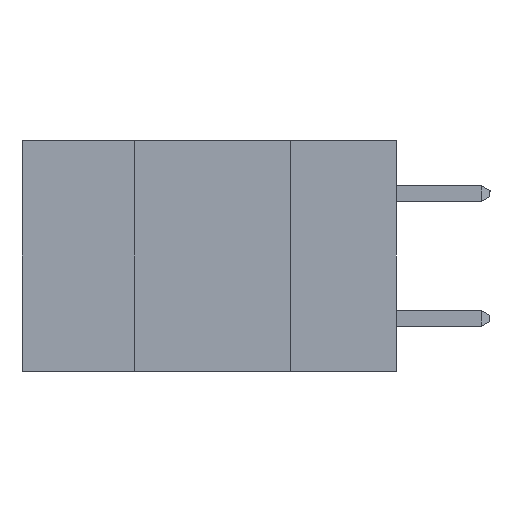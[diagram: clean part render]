
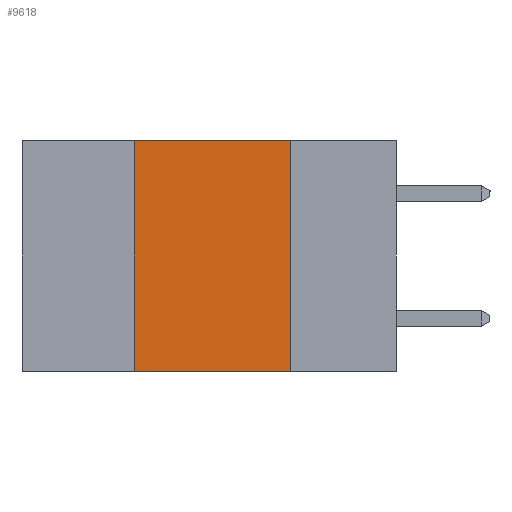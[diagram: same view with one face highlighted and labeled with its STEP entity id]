
A CAD part, left-side view. The second image highlights one B-rep face of the part: STEP entity #9618.
In plain terms, the highlighted planar face has unit normal (-1, 0, 0).
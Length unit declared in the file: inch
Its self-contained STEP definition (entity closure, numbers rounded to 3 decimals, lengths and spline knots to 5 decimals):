
#671 = VERTEX_POINT ( 'NONE', #12134 ) ;
#997 = FACE_OUTER_BOUND ( 'NONE', #4596, .T. ) ;
#1128 = EDGE_CURVE ( 'NONE', #8551, #1817, #10990, .T. ) ;
#1303 = ORIENTED_EDGE ( 'NONE', *, *, #12067, .F. ) ;
#1817 = VERTEX_POINT ( 'NONE', #8210 ) ;
#1913 = VERTEX_POINT ( 'NONE', #12137 ) ;
#2540 = DIRECTION ( 'NONE',  ( 0., 0., -1. ) ) ;
#2556 = EDGE_CURVE ( 'NONE', #671, #1913, #8167, .T. ) ;
#2598 = LINE ( 'NONE', #8309, #9945 ) ;
#4596 = EDGE_LOOP ( 'NONE', ( #7938, #5382, #1303, #8873 ) ) ;
#4763 = DIRECTION ( 'NONE',  ( 0., -1., 0. ) ) ;
#4802 = PLANE ( 'NONE',  #6367 ) ;
#4864 = DIRECTION ( 'NONE',  ( 1., 0., 0. ) ) ;
#5376 = CARTESIAN_POINT ( 'NONE',  ( 0., 0.6, -0.37 ) ) ;
#5382 = ORIENTED_EDGE ( 'NONE', *, *, #1128, .F. ) ;
#6367 = AXIS2_PLACEMENT_3D ( 'NONE', #8585, #4864, #9577 ) ;
#7640 = CARTESIAN_POINT ( 'NONE',  ( 0., 0.42, -0.37 ) ) ;
#7891 = DIRECTION ( 'NONE',  ( 0., 0., 1. ) ) ;
#7938 = ORIENTED_EDGE ( 'NONE', *, *, #10925, .F. ) ;
#8167 = LINE ( 'NONE', #5376, #10808 ) ;
#8210 = CARTESIAN_POINT ( 'NONE',  ( 0., 0.17, 0. ) ) ;
#8309 = CARTESIAN_POINT ( 'NONE',  ( 0., 0.17, -0.37 ) ) ;
#8484 = CARTESIAN_POINT ( 'NONE',  ( 0., 0.6, 0. ) ) ;
#8551 = VERTEX_POINT ( 'NONE', #9122 ) ;
#8585 = CARTESIAN_POINT ( 'NONE',  ( 0., 0.6, 0. ) ) ;
#8816 = LINE ( 'NONE', #7640, #10751 ) ;
#8873 = ORIENTED_EDGE ( 'NONE', *, *, #2556, .T. ) ;
#9122 = CARTESIAN_POINT ( 'NONE',  ( 0., 0.42, 0. ) ) ;
#9518 = VECTOR ( 'NONE', #4763, 39.37008 ) ;
#9577 = DIRECTION ( 'NONE',  ( 0., 0., -1. ) ) ;
#9618 = ADVANCED_FACE ( 'NONE', ( #997 ), #4802, .F. ) ;
#9945 = VECTOR ( 'NONE', #2540, 39.37008 ) ;
#10751 = VECTOR ( 'NONE', #7891, 39.37008 ) ;
#10808 = VECTOR ( 'NONE', #11972, 39.37008 ) ;
#10925 = EDGE_CURVE ( 'NONE', #1817, #1913, #2598, .T. ) ;
#10990 = LINE ( 'NONE', #8484, #9518 ) ;
#11972 = DIRECTION ( 'NONE',  ( 0., -1., 0. ) ) ;
#12067 = EDGE_CURVE ( 'NONE', #671, #8551, #8816, .T. ) ;
#12134 = CARTESIAN_POINT ( 'NONE',  ( 0., 0.42, -0.37 ) ) ;
#12137 = CARTESIAN_POINT ( 'NONE',  ( 0., 0.17, -0.37 ) ) ;
